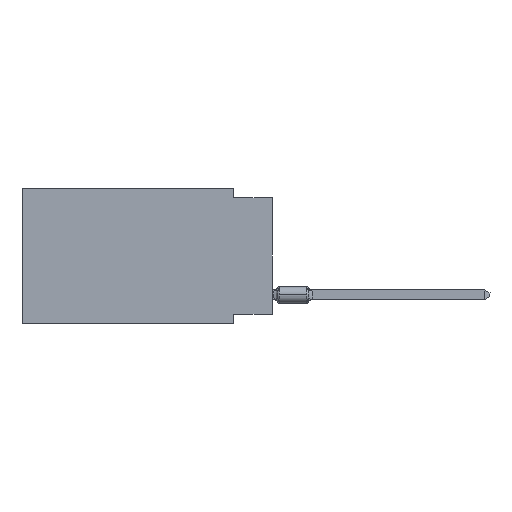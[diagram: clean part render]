
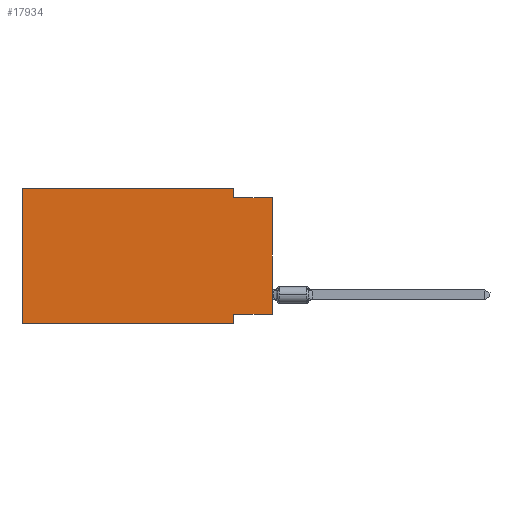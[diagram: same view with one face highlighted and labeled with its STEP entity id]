
A CAD part, left-side view. The second image highlights one B-rep face of the part: STEP entity #17934.
In plain terms, the highlighted planar face has unit normal (-1, 0, 0).
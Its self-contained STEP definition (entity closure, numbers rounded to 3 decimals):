
#425 = LINE ( 'NONE', #13262, #17444 ) ;
#527 = CARTESIAN_POINT ( 'NONE',  ( 0., 16.383, 0. ) ) ;
#982 = CARTESIAN_POINT ( 'NONE',  ( 0., 16.383, -8.89 ) ) ;
#1100 = VERTEX_POINT ( 'NONE', #21773 ) ;
#1368 = EDGE_CURVE ( 'NONE', #18464, #20310, #12544, .T. ) ;
#1854 = ORIENTED_EDGE ( 'NONE', *, *, #18607, .F. ) ;
#2117 = VECTOR ( 'NONE', #18677, 1000. ) ;
#2472 = DIRECTION ( 'NONE',  ( 0., -1., 0. ) ) ;
#2788 = CARTESIAN_POINT ( 'NONE',  ( 0., 16.383, 0. ) ) ;
#3009 = CARTESIAN_POINT ( 'NONE',  ( 0., 2.54, -8.89 ) ) ;
#3476 = ORIENTED_EDGE ( 'NONE', *, *, #12483, .F. ) ;
#5125 = DIRECTION ( 'NONE',  ( 0., 1., 0. ) ) ;
#5517 = LINE ( 'NONE', #18320, #2117 ) ;
#5662 = CARTESIAN_POINT ( 'NONE',  ( 0., 0., -0.635 ) ) ;
#5847 = ORIENTED_EDGE ( 'NONE', *, *, #1368, .F. ) ;
#6663 = LINE ( 'NONE', #3009, #12948 ) ;
#6777 = ORIENTED_EDGE ( 'NONE', *, *, #18806, .T. ) ;
#6881 = EDGE_CURVE ( 'NONE', #18538, #10543, #5517, .T. ) ;
#6991 = CARTESIAN_POINT ( 'NONE',  ( 0., 2.54, -0.635 ) ) ;
#7114 = LINE ( 'NONE', #16061, #13934 ) ;
#7565 = ORIENTED_EDGE ( 'NONE', *, *, #23358, .F. ) ;
#7937 = VECTOR ( 'NONE', #5125, 1000. ) ;
#8221 = VERTEX_POINT ( 'NONE', #9286 ) ;
#8370 = VERTEX_POINT ( 'NONE', #17488 ) ;
#8512 = FACE_OUTER_BOUND ( 'NONE', #17826, .T. ) ;
#8585 = VECTOR ( 'NONE', #11237, 1000. ) ;
#8586 = CARTESIAN_POINT ( 'NONE',  ( 0., 2.54, 0. ) ) ;
#8875 = VERTEX_POINT ( 'NONE', #19809 ) ;
#9286 = CARTESIAN_POINT ( 'NONE',  ( 0., 0., -8.255 ) ) ;
#9290 = ORIENTED_EDGE ( 'NONE', *, *, #6881, .F. ) ;
#10192 = DIRECTION ( 'NONE',  ( 0., 0., -1. ) ) ;
#10312 = EDGE_CURVE ( 'NONE', #18538, #8370, #22996, .T. ) ;
#10416 = DIRECTION ( 'NONE',  ( 0., 0., -1. ) ) ;
#10543 = VERTEX_POINT ( 'NONE', #527 ) ;
#11237 = DIRECTION ( 'NONE',  ( 0., -1., 0. ) ) ;
#11514 = ORIENTED_EDGE ( 'NONE', *, *, #10312, .T. ) ;
#12483 = EDGE_CURVE ( 'NONE', #8875, #8370, #6663, .T. ) ;
#12544 = LINE ( 'NONE', #8586, #19230 ) ;
#12948 = VECTOR ( 'NONE', #10416, 1000. ) ;
#13262 = CARTESIAN_POINT ( 'NONE',  ( 0., 16.383, 0. ) ) ;
#13934 = VECTOR ( 'NONE', #21737, 1000. ) ;
#14546 = CARTESIAN_POINT ( 'NONE',  ( 0., 0., -8.255 ) ) ;
#14692 = AXIS2_PLACEMENT_3D ( 'NONE', #2788, #19364, #10192 ) ;
#14848 = LINE ( 'NONE', #5662, #8585 ) ;
#15735 = ORIENTED_EDGE ( 'NONE', *, *, #15763, .F. ) ;
#15763 = EDGE_CURVE ( 'NONE', #8221, #8875, #21689, .T. ) ;
#16055 = DIRECTION ( 'NONE',  ( 0., 0., -1. ) ) ;
#16061 = CARTESIAN_POINT ( 'NONE',  ( 0., 0., 0. ) ) ;
#16168 = VECTOR ( 'NONE', #22875, 1000. ) ;
#17444 = VECTOR ( 'NONE', #2472, 1000. ) ;
#17488 = CARTESIAN_POINT ( 'NONE',  ( 0., 2.54, -8.89 ) ) ;
#17826 = EDGE_LOOP ( 'NONE', ( #6777, #1854, #5847, #7565, #9290, #11514, #3476, #15735 ) ) ;
#17934 = ADVANCED_FACE ( 'NONE', ( #8512 ), #23116, .F. ) ;
#18135 = CARTESIAN_POINT ( 'NONE',  ( 0., 2.54, 0. ) ) ;
#18320 = CARTESIAN_POINT ( 'NONE',  ( 0., 16.383, 0. ) ) ;
#18464 = VERTEX_POINT ( 'NONE', #18135 ) ;
#18538 = VERTEX_POINT ( 'NONE', #20636 ) ;
#18607 = EDGE_CURVE ( 'NONE', #20310, #1100, #14848, .T. ) ;
#18677 = DIRECTION ( 'NONE',  ( 0., 0., 1. ) ) ;
#18806 = EDGE_CURVE ( 'NONE', #8221, #1100, #7114, .T. ) ;
#19230 = VECTOR ( 'NONE', #16055, 1000. ) ;
#19364 = DIRECTION ( 'NONE',  ( 1., 0., 0. ) ) ;
#19809 = CARTESIAN_POINT ( 'NONE',  ( 0., 2.54, -8.255 ) ) ;
#20310 = VERTEX_POINT ( 'NONE', #6991 ) ;
#20636 = CARTESIAN_POINT ( 'NONE',  ( 0., 16.383, -8.89 ) ) ;
#21689 = LINE ( 'NONE', #14546, #7937 ) ;
#21737 = DIRECTION ( 'NONE',  ( 0., 0., 1. ) ) ;
#21773 = CARTESIAN_POINT ( 'NONE',  ( 0., 0., -0.635 ) ) ;
#22875 = DIRECTION ( 'NONE',  ( 0., -1., 0. ) ) ;
#22996 = LINE ( 'NONE', #982, #16168 ) ;
#23116 = PLANE ( 'NONE',  #14692 ) ;
#23358 = EDGE_CURVE ( 'NONE', #10543, #18464, #425, .T. ) ;
